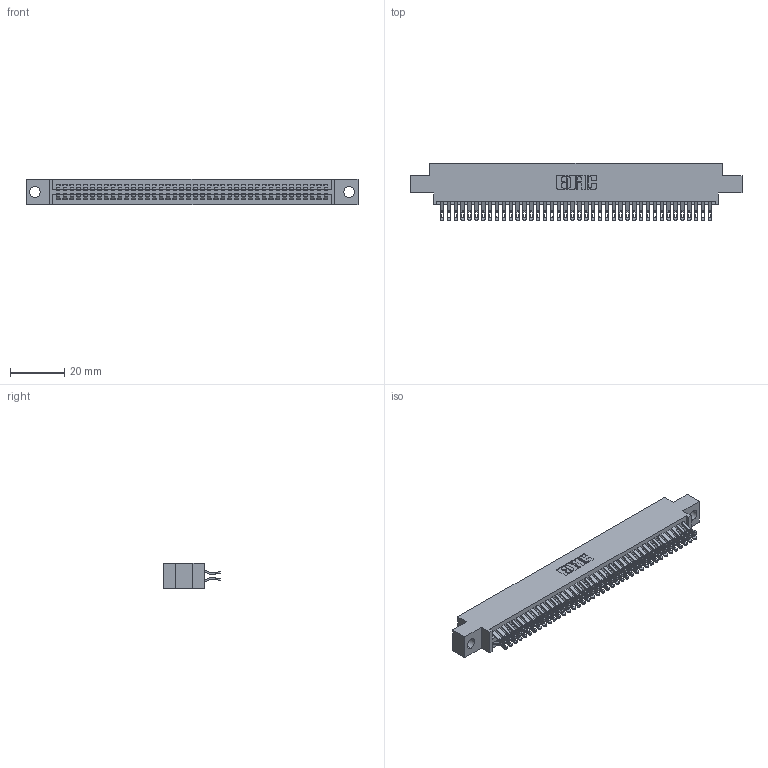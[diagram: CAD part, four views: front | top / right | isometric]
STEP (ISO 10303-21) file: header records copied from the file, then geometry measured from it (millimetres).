
FILE_DESCRIPTION (( 'STEP AP203' ), '1' );
FILE_NAME ('395-080-555-804.STEP', '2021-06-17T07:18:21', ( '' ), ( '' ), 'SwSTEP 2.0', 'SolidWorks 2020', '' );
FILE_SCHEMA (( 'CONFIG_CONTROL_DESIGN' ));
Length unit declared in the file: inch
Products named in the file (3): 395-080-555-804; 345-292-001_555 Tail; 345 Part_0.170 Offset - 0.156 Dia-TI
Assembly tree (81 placements, depth 2):
  395-080-555-804
    345 Part_0.170 Offset - 0.156 Dia-TI
    345-292-001_555 Tail  x80
Bounding box: 122.81 x 21.13 x 9.4 mm (x, y, z)
Volume: 11923.9 mm3; surface area: 18389 mm2
Topology: 81 solids, 81 shells, 4624 faces, 14549 edges, 9698 vertices
Faces by surface type: plane 2578, cylinder 2046
Entity records: 32531 total; most frequent: CARTESIAN_POINT 5496, ORIENTED_EDGE 5398, DIRECTION 4815, EDGE_CURVE 2699, VECTOR 2387, LINE 2387, VERTEX_POINT 1798, AXIS2_PLACEMENT_3D 1214
